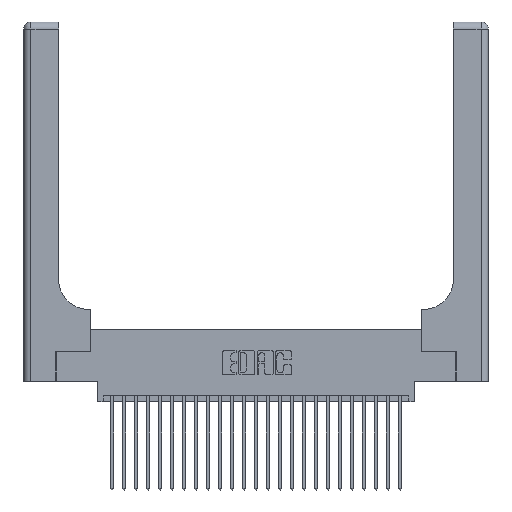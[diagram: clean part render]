
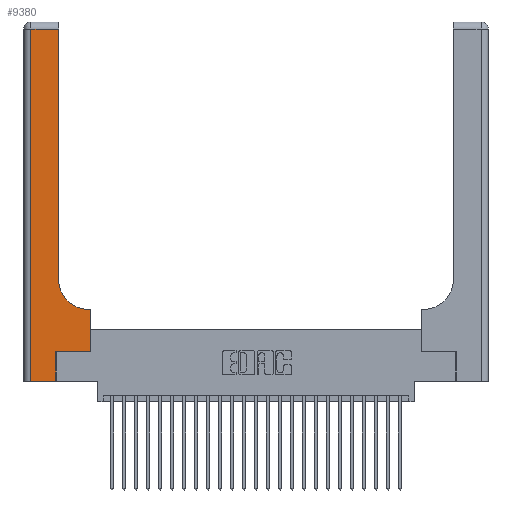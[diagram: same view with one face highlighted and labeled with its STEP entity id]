
A CAD part, top view. The second image highlights one B-rep face of the part: STEP entity #9380.
In plain terms, the highlighted planar face has unit normal (0, 0, 1).
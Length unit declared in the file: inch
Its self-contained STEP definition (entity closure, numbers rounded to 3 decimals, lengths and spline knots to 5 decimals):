
#100 = LINE ( 'NONE', #5146, #13623 ) ;
#240 = LINE ( 'NONE', #8818, #23300 ) ;
#1758 = VECTOR ( 'NONE', #1905, 39.37008 ) ;
#1905 = DIRECTION ( 'NONE',  ( 0., 1., 0. ) ) ;
#2165 = VERTEX_POINT ( 'NONE', #23885 ) ;
#2220 = EDGE_CURVE ( 'NONE', #21974, #4714, #100, .T. ) ;
#2556 = AXIS2_PLACEMENT_3D ( 'NONE', #4259, #25328, #12740 ) ;
#2953 = CARTESIAN_POINT ( 'NONE',  ( 0.2915, 0.6, 0.37 ) ) ;
#3096 = CARTESIAN_POINT ( 'NONE',  ( 0.06, 3., 0.37 ) ) ;
#3126 = CARTESIAN_POINT ( 'NONE',  ( 0.269, 0.25, 0.37 ) ) ;
#3913 = CARTESIAN_POINT ( 'NONE',  ( 0.5585, 0.25, 0.37 ) ) ;
#4259 = CARTESIAN_POINT ( 'NONE',  ( 0., 3., 0.37 ) ) ;
#4530 = VECTOR ( 'NONE', #17882, 39.37008 ) ;
#4714 = VERTEX_POINT ( 'NONE', #24954 ) ;
#5095 = VERTEX_POINT ( 'NONE', #21990 ) ;
#5146 = CARTESIAN_POINT ( 'NONE',  ( 0.2915, 3., 0.37 ) ) ;
#5415 = EDGE_CURVE ( 'NONE', #12074, #8326, #8701, .T. ) ;
#5664 = EDGE_CURVE ( 'NONE', #14444, #2165, #7032, .T. ) ;
#5925 = VERTEX_POINT ( 'NONE', #3913 ) ;
#7032 = LINE ( 'NONE', #3096, #23801 ) ;
#7454 = CARTESIAN_POINT ( 'NONE',  ( 0.5585, 0.6, 0.37 ) ) ;
#7563 = EDGE_CURVE ( 'NONE', #23779, #5095, #8907, .T. ) ;
#8114 = CARTESIAN_POINT ( 'NONE',  ( 0.2915, 0.85, 0.37 ) ) ;
#8122 = LINE ( 'NONE', #19068, #19312 ) ;
#8326 = VERTEX_POINT ( 'NONE', #24192 ) ;
#8502 = PLANE ( 'NONE',  #2556 ) ;
#8701 = LINE ( 'NONE', #10333, #1758 ) ;
#8813 = EDGE_CURVE ( 'NONE', #4714, #14444, #240, .T. ) ;
#8818 = CARTESIAN_POINT ( 'NONE',  ( 0., 2.94, 0.37 ) ) ;
#8907 = LINE ( 'NONE', #2953, #13181 ) ;
#9380 = ADVANCED_FACE ( 'NONE', ( #20004 ), #8502, .F. ) ;
#10333 = CARTESIAN_POINT ( 'NONE',  ( 0.269, 0., 0.37 ) ) ;
#11058 = LINE ( 'NONE', #16582, #27150 ) ;
#11193 = ORIENTED_EDGE ( 'NONE', *, *, #7563, .T. ) ;
#11231 = ORIENTED_EDGE ( 'NONE', *, *, #14214, .T. ) ;
#11992 = ORIENTED_EDGE ( 'NONE', *, *, #5664, .T. ) ;
#12074 = VERTEX_POINT ( 'NONE', #13954 ) ;
#12379 = DIRECTION ( 'NONE',  ( 0., 0., -1. ) ) ;
#12723 = DIRECTION ( 'NONE',  ( 1., 0., 0. ) ) ;
#12740 = DIRECTION ( 'NONE',  ( -1., 0., 0. ) ) ;
#13098 = LINE ( 'NONE', #3126, #4530 ) ;
#13181 = VECTOR ( 'NONE', #24023, 39.37008 ) ;
#13259 = CARTESIAN_POINT ( 'NONE',  ( 0.06, 2.94, 0.37 ) ) ;
#13623 = VECTOR ( 'NONE', #26191, 39.37008 ) ;
#13954 = CARTESIAN_POINT ( 'NONE',  ( 0.269, 0., 0.37 ) ) ;
#14214 = EDGE_CURVE ( 'NONE', #2165, #12074, #8122, .T. ) ;
#14444 = VERTEX_POINT ( 'NONE', #13259 ) ;
#14452 = DIRECTION ( 'NONE',  ( 0., 1., 0. ) ) ;
#14816 = EDGE_CURVE ( 'NONE', #5925, #23779, #11058, .T. ) ;
#15420 = ORIENTED_EDGE ( 'NONE', *, *, #20878, .T. ) ;
#15670 = ORIENTED_EDGE ( 'NONE', *, *, #14816, .T. ) ;
#16582 = CARTESIAN_POINT ( 'NONE',  ( 0.5585, 0.25, 0.37 ) ) ;
#16918 = ORIENTED_EDGE ( 'NONE', *, *, #21367, .T. ) ;
#17351 = CIRCLE ( 'NONE', #18624, 0.25 ) ;
#17882 = DIRECTION ( 'NONE',  ( 1., 0., 0. ) ) ;
#18624 = AXIS2_PLACEMENT_3D ( 'NONE', #24956, #12379, #27061 ) ;
#18844 = ORIENTED_EDGE ( 'NONE', *, *, #2220, .T. ) ;
#19068 = CARTESIAN_POINT ( 'NONE',  ( 0., 0., 0.37 ) ) ;
#19312 = VECTOR ( 'NONE', #12723, 39.37008 ) ;
#20004 = FACE_OUTER_BOUND ( 'NONE', #20256, .T. ) ;
#20256 = EDGE_LOOP ( 'NONE', ( #18844, #24545, #11992, #11231, #23096, #15420, #15670, #11193, #16918 ) ) ;
#20878 = EDGE_CURVE ( 'NONE', #8326, #5925, #13098, .T. ) ;
#21367 = EDGE_CURVE ( 'NONE', #5095, #21974, #17351, .T. ) ;
#21397 = DIRECTION ( 'NONE',  ( -1., 0., 0. ) ) ;
#21974 = VERTEX_POINT ( 'NONE', #8114 ) ;
#21990 = CARTESIAN_POINT ( 'NONE',  ( 0.5415, 0.6, 0.37 ) ) ;
#23096 = ORIENTED_EDGE ( 'NONE', *, *, #5415, .T. ) ;
#23300 = VECTOR ( 'NONE', #21397, 39.37008 ) ;
#23779 = VERTEX_POINT ( 'NONE', #7454 ) ;
#23801 = VECTOR ( 'NONE', #24172, 39.37008 ) ;
#23885 = CARTESIAN_POINT ( 'NONE',  ( 0.06, 0., 0.37 ) ) ;
#24023 = DIRECTION ( 'NONE',  ( -1., 0., 0. ) ) ;
#24172 = DIRECTION ( 'NONE',  ( 0., -1., 0. ) ) ;
#24192 = CARTESIAN_POINT ( 'NONE',  ( 0.269, 0.25, 0.37 ) ) ;
#24545 = ORIENTED_EDGE ( 'NONE', *, *, #8813, .T. ) ;
#24954 = CARTESIAN_POINT ( 'NONE',  ( 0.2915, 2.94, 0.37 ) ) ;
#24956 = CARTESIAN_POINT ( 'NONE',  ( 0.5415, 0.85, 0.37 ) ) ;
#25328 = DIRECTION ( 'NONE',  ( 0., 0., -1. ) ) ;
#26191 = DIRECTION ( 'NONE',  ( 0., 1., 0. ) ) ;
#27061 = DIRECTION ( 'NONE',  ( 1., 0., 0. ) ) ;
#27150 = VECTOR ( 'NONE', #14452, 39.37008 ) ;
